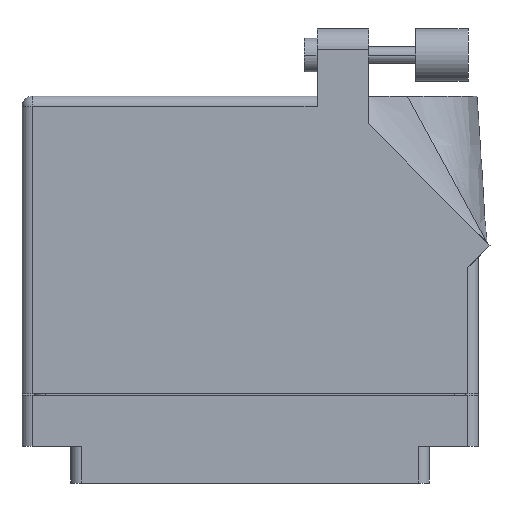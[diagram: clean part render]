
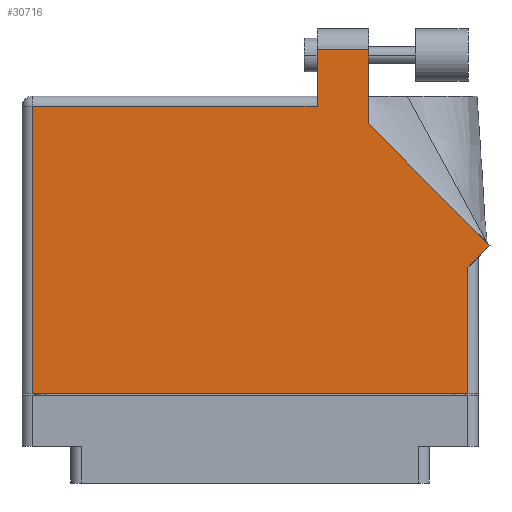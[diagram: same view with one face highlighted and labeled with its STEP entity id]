
A CAD part, front view. The second image highlights one B-rep face of the part: STEP entity #30716.
In plain terms, the highlighted face is planar.
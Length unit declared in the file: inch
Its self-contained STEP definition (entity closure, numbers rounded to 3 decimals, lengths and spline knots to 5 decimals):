
#113 = VECTOR ( 'NONE', #48751, 39.37008 ) ;
#274 = ORIENTED_EDGE ( 'NONE', *, *, #64345, .T. ) ;
#2877 = VERTEX_POINT ( 'NONE', #57672 ) ;
#3059 = VECTOR ( 'NONE', #58655, 39.37008 ) ;
#3928 = CARTESIAN_POINT ( 'NONE',  ( -1.359, 1.675, 0.617 ) ) ;
#4582 = DIRECTION ( 'NONE',  ( 0., 1., 0. ) ) ;
#5034 = VERTEX_POINT ( 'NONE', #32740 ) ;
#5848 = CARTESIAN_POINT ( 'NONE',  ( 0.706, 1.50942, 0.617 ) ) ;
#6676 = ORIENTED_EDGE ( 'NONE', *, *, #55890, .T. ) ;
#9580 = CARTESIAN_POINT ( 'NONE',  ( -1.297, -0.1, 0.617 ) ) ;
#12902 = CARTESIAN_POINT ( 'NONE',  ( 1.297, -0.1, 0.617 ) ) ;
#13161 = LINE ( 'NONE', #34505, #64709 ) ;
#13606 = LINE ( 'NONE', #36374, #15902 ) ;
#13997 = EDGE_CURVE ( 'NONE', #53167, #18525, #22787, .T. ) ;
#14634 = EDGE_LOOP ( 'NONE', ( #26137, #22809, #63707, #44889, #19286, #6676, #48200, #17426, #274 ) ) ;
#15210 = VECTOR ( 'NONE', #20104, 39.37008 ) ;
#15697 = EDGE_CURVE ( 'NONE', #34993, #54075, #13161, .T. ) ;
#15826 = DIRECTION ( 'NONE',  ( -0.707, 0.707, 0. ) ) ;
#15902 = VECTOR ( 'NONE', #15826, 39.37008 ) ;
#17426 = ORIENTED_EDGE ( 'NONE', *, *, #48419, .T. ) ;
#18525 = VERTEX_POINT ( 'NONE', #37131 ) ;
#19286 = ORIENTED_EDGE ( 'NONE', *, *, #59787, .T. ) ;
#19902 = VECTOR ( 'NONE', #27881, 39.37008 ) ;
#20104 = DIRECTION ( 'NONE',  ( -1., 0., 0. ) ) ;
#21259 = CARTESIAN_POINT ( 'NONE',  ( 1.297, 0.653, 0.617 ) ) ;
#22787 = LINE ( 'NONE', #62492, #113 ) ;
#22809 = ORIENTED_EDGE ( 'NONE', *, *, #13997, .T. ) ;
#23211 = LINE ( 'NONE', #52638, #62350 ) ;
#23700 = CARTESIAN_POINT ( 'NONE',  ( 1.359, 0.715, 0.617 ) ) ;
#24481 = LINE ( 'NONE', #37897, #36166 ) ;
#24795 = VERTEX_POINT ( 'NONE', #41151 ) ;
#26123 = EDGE_CURVE ( 'NONE', #18525, #24795, #23211, .T. ) ;
#26137 = ORIENTED_EDGE ( 'NONE', *, *, #58388, .T. ) ;
#27881 = DIRECTION ( 'NONE',  ( 0.707, 0.707, 0. ) ) ;
#29844 = CARTESIAN_POINT ( 'NONE',  ( 0.706, 1.95, 0.617 ) ) ;
#30034 = VECTOR ( 'NONE', #35772, 39.37008 ) ;
#30716 = ADVANCED_FACE ( 'NONE', ( #31255 ), #49592, .F. ) ;
#31255 = FACE_OUTER_BOUND ( 'NONE', #14634, .T. ) ;
#32740 = CARTESIAN_POINT ( 'NONE',  ( 0.706, 1.50942, 0.617 ) ) ;
#34505 = CARTESIAN_POINT ( 'NONE',  ( 1.297, 0.715, 0.617 ) ) ;
#34806 = CARTESIAN_POINT ( 'NONE',  ( -1.359, 1.613, 0.617 ) ) ;
#34993 = VERTEX_POINT ( 'NONE', #12902 ) ;
#35772 = DIRECTION ( 'NONE',  ( 0., 1., 0. ) ) ;
#36166 = VECTOR ( 'NONE', #42946, 39.37008 ) ;
#36374 = CARTESIAN_POINT ( 'NONE',  ( 1.42971, 0.78571, 0.617 ) ) ;
#37131 = CARTESIAN_POINT ( 'NONE',  ( 0.399, 1.95, 0.617 ) ) ;
#37716 = CARTESIAN_POINT ( 'NONE',  ( -1.297, 1.613, 0.617 ) ) ;
#37802 = DIRECTION ( 'NONE',  ( 0., -1., 0. ) ) ;
#37897 = CARTESIAN_POINT ( 'NONE',  ( -1.297, -0.1, 0.617 ) ) ;
#39070 = DIRECTION ( 'NONE',  ( -1., 0., 0. ) ) ;
#41151 = CARTESIAN_POINT ( 'NONE',  ( 0.399, 1.613, 0.617 ) ) ;
#41865 = LINE ( 'NONE', #34806, #15210 ) ;
#42946 = DIRECTION ( 'NONE',  ( 0., -1., 0. ) ) ;
#44889 = ORIENTED_EDGE ( 'NONE', *, *, #63599, .T. ) ;
#46439 = VERTEX_POINT ( 'NONE', #37716 ) ;
#48171 = LINE ( 'NONE', #23700, #19902 ) ;
#48200 = ORIENTED_EDGE ( 'NONE', *, *, #15697, .T. ) ;
#48419 = EDGE_CURVE ( 'NONE', #54075, #2877, #48171, .T. ) ;
#48751 = DIRECTION ( 'NONE',  ( -1., 0., 0. ) ) ;
#48838 = LINE ( 'NONE', #5848, #30034 ) ;
#49592 = PLANE ( 'NONE',  #61663 ) ;
#52638 = CARTESIAN_POINT ( 'NONE',  ( 0.399, 1.675, 0.617 ) ) ;
#53167 = VERTEX_POINT ( 'NONE', #29844 ) ;
#53246 = CARTESIAN_POINT ( 'NONE',  ( -1.359, -0.1, 0.617 ) ) ;
#54075 = VERTEX_POINT ( 'NONE', #21259 ) ;
#54131 = DIRECTION ( 'NONE',  ( 0., 0., -1. ) ) ;
#55890 = EDGE_CURVE ( 'NONE', #63204, #34993, #63220, .T. ) ;
#57672 = CARTESIAN_POINT ( 'NONE',  ( 1.42971, 0.78571, 0.617 ) ) ;
#58388 = EDGE_CURVE ( 'NONE', #5034, #53167, #48838, .T. ) ;
#58655 = DIRECTION ( 'NONE',  ( 1., 0., 0. ) ) ;
#59787 = EDGE_CURVE ( 'NONE', #46439, #63204, #24481, .T. ) ;
#61663 = AXIS2_PLACEMENT_3D ( 'NONE', #3928, #54131, #39070 ) ;
#62350 = VECTOR ( 'NONE', #37802, 39.37008 ) ;
#62492 = CARTESIAN_POINT ( 'NONE',  ( 0.399, 1.95, 0.617 ) ) ;
#63204 = VERTEX_POINT ( 'NONE', #9580 ) ;
#63220 = LINE ( 'NONE', #53246, #3059 ) ;
#63599 = EDGE_CURVE ( 'NONE', #24795, #46439, #41865, .T. ) ;
#63707 = ORIENTED_EDGE ( 'NONE', *, *, #26123, .T. ) ;
#64345 = EDGE_CURVE ( 'NONE', #2877, #5034, #13606, .T. ) ;
#64709 = VECTOR ( 'NONE', #4582, 39.37008 ) ;
